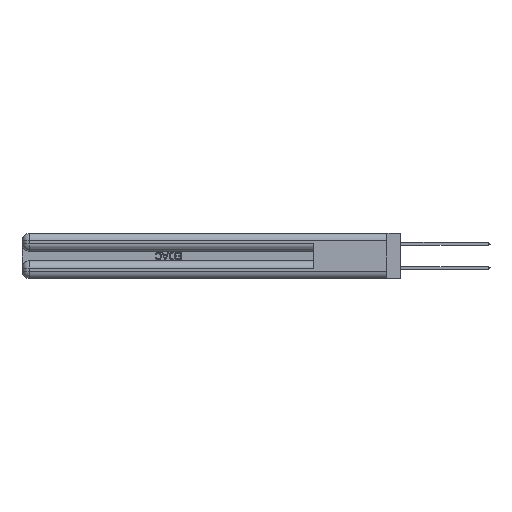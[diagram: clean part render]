
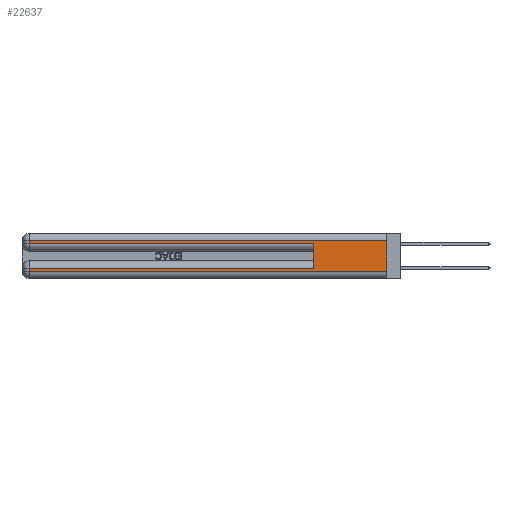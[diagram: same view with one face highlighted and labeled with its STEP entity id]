
A CAD part, left-side view. The second image highlights one B-rep face of the part: STEP entity #22637.
In plain terms, the highlighted planar face has unit normal (-1, 0, 0).
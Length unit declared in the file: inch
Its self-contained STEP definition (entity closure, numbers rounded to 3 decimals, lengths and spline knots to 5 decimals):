
#191 = VERTEX_POINT ( 'NONE', #36442 ) ;
#1212 = DIRECTION ( 'NONE',  ( 0., 0., -1. ) ) ;
#1363 = DIRECTION ( 'NONE',  ( 0., 1., 0. ) ) ;
#3113 = CARTESIAN_POINT ( 'NONE',  ( 0., 0., 0.06 ) ) ;
#3925 = AXIS2_PLACEMENT_3D ( 'NONE', #9484, #16762, #41845 ) ;
#4003 = DIRECTION ( 'NONE',  ( 0., 0., -1. ) ) ;
#6327 = EDGE_CURVE ( 'NONE', #39035, #37482, #43671, .T. ) ;
#6407 = VECTOR ( 'NONE', #13685, 39.37008 ) ;
#6685 = EDGE_CURVE ( 'NONE', #7961, #13172, #20228, .T. ) ;
#7230 = EDGE_CURVE ( 'NONE', #24170, #32637, #33671, .T. ) ;
#7961 = VERTEX_POINT ( 'NONE', #18299 ) ;
#8691 = EDGE_CURVE ( 'NONE', #191, #44716, #24678, .T. ) ;
#9484 = CARTESIAN_POINT ( 'NONE',  ( 0., 0., 0.37 ) ) ;
#10835 = FACE_OUTER_BOUND ( 'NONE', #21657, .T. ) ;
#11996 = CARTESIAN_POINT ( 'NONE',  ( 0., 2.94, 0.37 ) ) ;
#12100 = EDGE_CURVE ( 'NONE', #24170, #39035, #26035, .T. ) ;
#12753 = LINE ( 'NONE', #3113, #29669 ) ;
#12970 = PLANE ( 'NONE',  #3925 ) ;
#13172 = VERTEX_POINT ( 'NONE', #38237 ) ;
#13685 = DIRECTION ( 'NONE',  ( 0., -1., 0. ) ) ;
#15243 = VECTOR ( 'NONE', #38918, 39.37008 ) ;
#16704 = CARTESIAN_POINT ( 'NONE',  ( 0., 2.94, 0.06 ) ) ;
#16762 = DIRECTION ( 'NONE',  ( 1., 0., 0. ) ) ;
#16966 = CARTESIAN_POINT ( 'NONE',  ( 0., 0.6, 0.085 ) ) ;
#17129 = CARTESIAN_POINT ( 'NONE',  ( 0., 0.6, 0.285 ) ) ;
#17406 = CARTESIAN_POINT ( 'NONE',  ( 0., 0., 0.085 ) ) ;
#18299 = CARTESIAN_POINT ( 'NONE',  ( 0., 2.94, 0.31 ) ) ;
#20228 = LINE ( 'NONE', #11996, #29797 ) ;
#21350 = EDGE_CURVE ( 'NONE', #13172, #32637, #35183, .T. ) ;
#21657 = EDGE_LOOP ( 'NONE', ( #30151, #33046, #25636, #30284, #25740, #28138, #33211, #28210 ) ) ;
#22637 = ADVANCED_FACE ( 'NONE', ( #10835 ), #12970, .F. ) ;
#23559 = VECTOR ( 'NONE', #4003, 39.37008 ) ;
#24170 = VERTEX_POINT ( 'NONE', #16966 ) ;
#24181 = VECTOR ( 'NONE', #29922, 39.37008 ) ;
#24678 = LINE ( 'NONE', #40039, #23559 ) ;
#25636 = ORIENTED_EDGE ( 'NONE', *, *, #6685, .T. ) ;
#25740 = ORIENTED_EDGE ( 'NONE', *, *, #7230, .F. ) ;
#26035 = LINE ( 'NONE', #17406, #15243 ) ;
#27516 = EDGE_CURVE ( 'NONE', #37482, #44716, #12753, .T. ) ;
#28138 = ORIENTED_EDGE ( 'NONE', *, *, #12100, .T. ) ;
#28210 = ORIENTED_EDGE ( 'NONE', *, *, #27516, .T. ) ;
#29669 = VECTOR ( 'NONE', #35617, 39.37008 ) ;
#29797 = VECTOR ( 'NONE', #1212, 39.37008 ) ;
#29922 = DIRECTION ( 'NONE',  ( 0., 0., 1. ) ) ;
#30151 = ORIENTED_EDGE ( 'NONE', *, *, #8691, .F. ) ;
#30284 = ORIENTED_EDGE ( 'NONE', *, *, #21350, .T. ) ;
#32637 = VERTEX_POINT ( 'NONE', #17129 ) ;
#33046 = ORIENTED_EDGE ( 'NONE', *, *, #37327, .T. ) ;
#33211 = ORIENTED_EDGE ( 'NONE', *, *, #6327, .T. ) ;
#33671 = LINE ( 'NONE', #40530, #24181 ) ;
#35183 = LINE ( 'NONE', #38857, #6407 ) ;
#35617 = DIRECTION ( 'NONE',  ( 0., -1., 0. ) ) ;
#36442 = CARTESIAN_POINT ( 'NONE',  ( 0., 0., 0.31 ) ) ;
#36690 = VECTOR ( 'NONE', #1363, 39.37008 ) ;
#37327 = EDGE_CURVE ( 'NONE', #191, #7961, #37796, .T. ) ;
#37482 = VERTEX_POINT ( 'NONE', #16704 ) ;
#37796 = LINE ( 'NONE', #44420, #36690 ) ;
#38237 = CARTESIAN_POINT ( 'NONE',  ( 0., 2.94, 0.285 ) ) ;
#38857 = CARTESIAN_POINT ( 'NONE',  ( 0., 0., 0.285 ) ) ;
#38918 = DIRECTION ( 'NONE',  ( 0., 1., 0. ) ) ;
#39035 = VERTEX_POINT ( 'NONE', #41313 ) ;
#40039 = CARTESIAN_POINT ( 'NONE',  ( 0., 0., 0.37 ) ) ;
#40530 = CARTESIAN_POINT ( 'NONE',  ( 0., 0.6, 0.145 ) ) ;
#41313 = CARTESIAN_POINT ( 'NONE',  ( 0., 2.94, 0.085 ) ) ;
#41845 = DIRECTION ( 'NONE',  ( 0., 0., -1. ) ) ;
#42300 = DIRECTION ( 'NONE',  ( 0., 0., -1. ) ) ;
#43193 = VECTOR ( 'NONE', #42300, 39.37008 ) ;
#43671 = LINE ( 'NONE', #45858, #43193 ) ;
#44420 = CARTESIAN_POINT ( 'NONE',  ( 0., 0., 0.31 ) ) ;
#44716 = VERTEX_POINT ( 'NONE', #46246 ) ;
#45858 = CARTESIAN_POINT ( 'NONE',  ( 0., 2.94, 0.37 ) ) ;
#46246 = CARTESIAN_POINT ( 'NONE',  ( 0., 0., 0.06 ) ) ;
